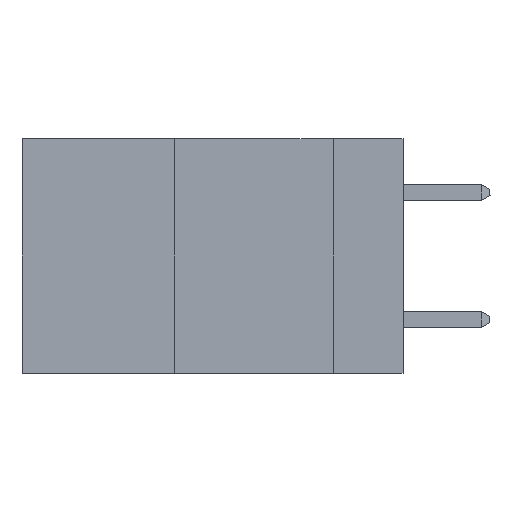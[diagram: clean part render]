
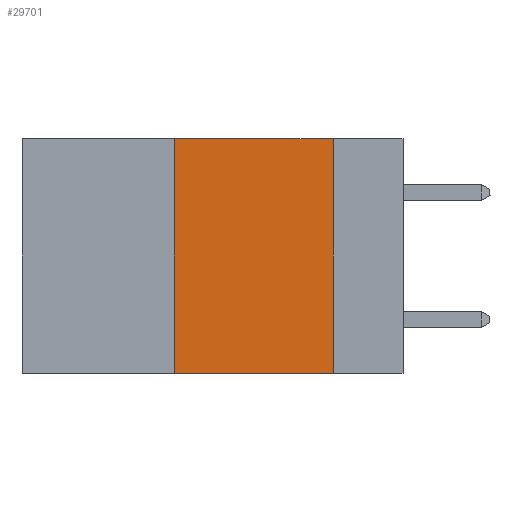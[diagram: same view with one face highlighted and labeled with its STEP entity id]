
A CAD part, left-side view. The second image highlights one B-rep face of the part: STEP entity #29701.
In plain terms, the highlighted planar face has unit normal (-1, 0, 0).
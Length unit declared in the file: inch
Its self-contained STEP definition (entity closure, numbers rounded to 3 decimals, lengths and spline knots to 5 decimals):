
#461 = ORIENTED_EDGE ( 'NONE', *, *, #23714, .F. ) ;
#1154 = EDGE_CURVE ( 'NONE', #2975, #19138, #23781, .T. ) ;
#1460 = ORIENTED_EDGE ( 'NONE', *, *, #6981, .T. ) ;
#2975 = VERTEX_POINT ( 'NONE', #7432 ) ;
#4202 = DIRECTION ( 'NONE',  ( 0., 0., 1. ) ) ;
#5187 = PLANE ( 'NONE',  #34133 ) ;
#6981 = EDGE_CURVE ( 'NONE', #30229, #25758, #19919, .T. ) ;
#7003 = LINE ( 'NONE', #18719, #15637 ) ;
#7432 = CARTESIAN_POINT ( 'NONE',  ( 0., 0.36, 0. ) ) ;
#7600 = DIRECTION ( 'NONE',  ( 0., 0., -1. ) ) ;
#14152 = CARTESIAN_POINT ( 'NONE',  ( 0., 0.11, 0. ) ) ;
#14506 = EDGE_LOOP ( 'NONE', ( #461, #19601, #26278, #1460 ) ) ;
#15637 = VECTOR ( 'NONE', #4202, 39.37008 ) ;
#16231 = EDGE_CURVE ( 'NONE', #30229, #2975, #7003, .T. ) ;
#17667 = DIRECTION ( 'NONE',  ( 0., -1., 0. ) ) ;
#18719 = CARTESIAN_POINT ( 'NONE',  ( 0., 0.36, 0. ) ) ;
#19136 = CARTESIAN_POINT ( 'NONE',  ( 0., 0.6, 0. ) ) ;
#19138 = VERTEX_POINT ( 'NONE', #14152 ) ;
#19601 = ORIENTED_EDGE ( 'NONE', *, *, #1154, .F. ) ;
#19919 = LINE ( 'NONE', #29012, #24216 ) ;
#23714 = EDGE_CURVE ( 'NONE', #19138, #25758, #25362, .T. ) ;
#23781 = LINE ( 'NONE', #24334, #23793 ) ;
#23793 = VECTOR ( 'NONE', #27305, 39.37008 ) ;
#24216 = VECTOR ( 'NONE', #17667, 39.37008 ) ;
#24334 = CARTESIAN_POINT ( 'NONE',  ( 0., 0.6, 0. ) ) ;
#25362 = LINE ( 'NONE', #36728, #35701 ) ;
#25758 = VERTEX_POINT ( 'NONE', #32931 ) ;
#26278 = ORIENTED_EDGE ( 'NONE', *, *, #16231, .F. ) ;
#27305 = DIRECTION ( 'NONE',  ( 0., -1., 0. ) ) ;
#27326 = DIRECTION ( 'NONE',  ( 1., 0., 0. ) ) ;
#27836 = CARTESIAN_POINT ( 'NONE',  ( 0., 0.36, -0.37 ) ) ;
#29012 = CARTESIAN_POINT ( 'NONE',  ( 0., 0.6, -0.37 ) ) ;
#29701 = ADVANCED_FACE ( 'NONE', ( #33092 ), #5187, .F. ) ;
#30229 = VERTEX_POINT ( 'NONE', #27836 ) ;
#31499 = DIRECTION ( 'NONE',  ( 0., 0., -1. ) ) ;
#32931 = CARTESIAN_POINT ( 'NONE',  ( 0., 0.11, -0.37 ) ) ;
#33092 = FACE_OUTER_BOUND ( 'NONE', #14506, .T. ) ;
#34133 = AXIS2_PLACEMENT_3D ( 'NONE', #19136, #27326, #7600 ) ;
#35701 = VECTOR ( 'NONE', #31499, 39.37008 ) ;
#36728 = CARTESIAN_POINT ( 'NONE',  ( 0., 0.11, 0. ) ) ;
